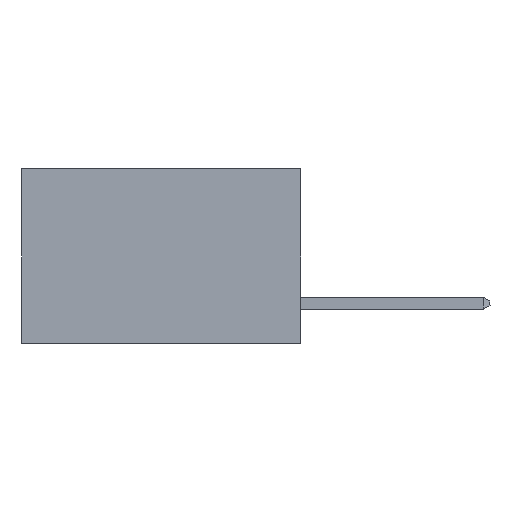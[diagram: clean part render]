
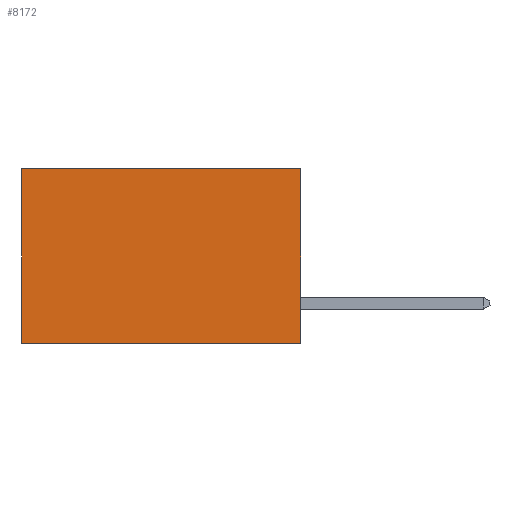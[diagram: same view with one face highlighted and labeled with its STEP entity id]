
A CAD part, left-side view. The second image highlights one B-rep face of the part: STEP entity #8172.
In plain terms, the highlighted planar face has unit normal (-1, 0, 0).
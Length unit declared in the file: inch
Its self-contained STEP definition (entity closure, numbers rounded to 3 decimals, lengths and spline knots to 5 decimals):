
#213 = AXIS2_PLACEMENT_3D ( 'NONE', #6247, #14322, #7424 ) ;
#350 = CARTESIAN_POINT ( 'NONE',  ( 0.277, 0.59, -0.37 ) ) ;
#540 = CARTESIAN_POINT ( 'NONE',  ( 0.277, 0., 0. ) ) ;
#1268 = VERTEX_POINT ( 'NONE', #13286 ) ;
#1470 = PLANE ( 'NONE',  #213 ) ;
#1758 = EDGE_CURVE ( 'NONE', #1268, #7723, #13324, .T. ) ;
#1924 = LINE ( 'NONE', #4738, #4764 ) ;
#1987 = DIRECTION ( 'NONE',  ( 0., 0., -1. ) ) ;
#2702 = EDGE_CURVE ( 'NONE', #11617, #1268, #9916, .T. ) ;
#3139 = CARTESIAN_POINT ( 'NONE',  ( 0.277, 0.59, -0.37 ) ) ;
#3576 = DIRECTION ( 'NONE',  ( 0., 1., 0. ) ) ;
#4312 = ORIENTED_EDGE ( 'NONE', *, *, #1758, .T. ) ;
#4387 = CARTESIAN_POINT ( 'NONE',  ( 0.277, 0., -0.37 ) ) ;
#4738 = CARTESIAN_POINT ( 'NONE',  ( 0.277, 0., -0.37 ) ) ;
#4764 = VECTOR ( 'NONE', #3576, 39.37008 ) ;
#4893 = ORIENTED_EDGE ( 'NONE', *, *, #13655, .F. ) ;
#5175 = CARTESIAN_POINT ( 'NONE',  ( 0.277, 0., -0.37 ) ) ;
#6247 = CARTESIAN_POINT ( 'NONE',  ( 0.277, 0., -0.37 ) ) ;
#7331 = VECTOR ( 'NONE', #14732, 39.37008 ) ;
#7424 = DIRECTION ( 'NONE',  ( 0., 0., -1. ) ) ;
#7723 = VERTEX_POINT ( 'NONE', #3139 ) ;
#7876 = VECTOR ( 'NONE', #1987, 39.37008 ) ;
#8172 = ADVANCED_FACE ( 'NONE', ( #13237 ), #1470, .F. ) ;
#9671 = EDGE_LOOP ( 'NONE', ( #4312, #4893, #12082, #10118 ) ) ;
#9916 = LINE ( 'NONE', #540, #12610 ) ;
#10118 = ORIENTED_EDGE ( 'NONE', *, *, #2702, .T. ) ;
#10612 = EDGE_CURVE ( 'NONE', #11617, #13919, #14190, .T. ) ;
#11617 = VERTEX_POINT ( 'NONE', #14781 ) ;
#12082 = ORIENTED_EDGE ( 'NONE', *, *, #10612, .F. ) ;
#12368 = DIRECTION ( 'NONE',  ( 0., 1., 0. ) ) ;
#12610 = VECTOR ( 'NONE', #12368, 39.37008 ) ;
#13237 = FACE_OUTER_BOUND ( 'NONE', #9671, .T. ) ;
#13286 = CARTESIAN_POINT ( 'NONE',  ( 0.277, 0.59, 0. ) ) ;
#13324 = LINE ( 'NONE', #350, #7876 ) ;
#13655 = EDGE_CURVE ( 'NONE', #13919, #7723, #1924, .T. ) ;
#13919 = VERTEX_POINT ( 'NONE', #5175 ) ;
#14190 = LINE ( 'NONE', #4387, #7331 ) ;
#14322 = DIRECTION ( 'NONE',  ( 1., 0., 0. ) ) ;
#14732 = DIRECTION ( 'NONE',  ( 0., 0., -1. ) ) ;
#14781 = CARTESIAN_POINT ( 'NONE',  ( 0.277, 0., 0. ) ) ;
